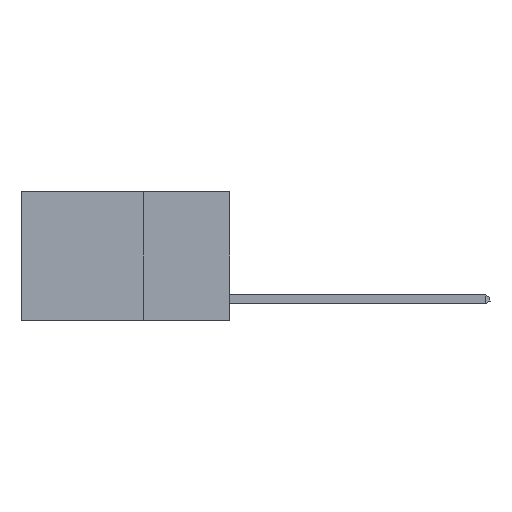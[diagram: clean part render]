
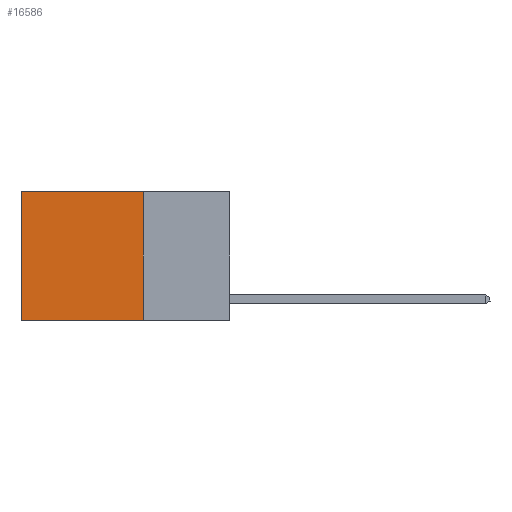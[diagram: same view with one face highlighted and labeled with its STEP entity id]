
A CAD part, left-side view. The second image highlights one B-rep face of the part: STEP entity #16586.
In plain terms, the highlighted planar face has unit normal (-1, 0, 0).
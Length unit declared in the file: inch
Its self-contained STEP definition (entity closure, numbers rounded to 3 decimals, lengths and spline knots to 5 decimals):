
#429 = VECTOR ( 'NONE', #10084, 39.37008 ) ;
#1538 = CARTESIAN_POINT ( 'NONE',  ( 0.2625, 0.25, -0.37 ) ) ;
#2339 = VERTEX_POINT ( 'NONE', #7589 ) ;
#2735 = AXIS2_PLACEMENT_3D ( 'NONE', #7296, #7208, #12312 ) ;
#3095 = LINE ( 'NONE', #10648, #5318 ) ;
#3541 = EDGE_CURVE ( 'NONE', #4128, #12841, #11182, .T. ) ;
#4128 = VERTEX_POINT ( 'NONE', #5209 ) ;
#4761 = LINE ( 'NONE', #4850, #5899 ) ;
#4764 = FACE_OUTER_BOUND ( 'NONE', #12498, .T. ) ;
#4850 = CARTESIAN_POINT ( 'NONE',  ( 0.2625, 0.25, -0.37 ) ) ;
#4935 = DIRECTION ( 'NONE',  ( 0., 0., -1. ) ) ;
#5209 = CARTESIAN_POINT ( 'NONE',  ( 0.2625, 0.6, 0. ) ) ;
#5318 = VECTOR ( 'NONE', #11742, 39.37008 ) ;
#5486 = ORIENTED_EDGE ( 'NONE', *, *, #15442, .F. ) ;
#5899 = VECTOR ( 'NONE', #16595, 39.37008 ) ;
#6091 = CARTESIAN_POINT ( 'NONE',  ( 0.2625, 0.6, -0.37 ) ) ;
#7208 = DIRECTION ( 'NONE',  ( 1., 0., 0. ) ) ;
#7264 = VECTOR ( 'NONE', #4935, 39.37008 ) ;
#7296 = CARTESIAN_POINT ( 'NONE',  ( 0.2625, 0.25, 0. ) ) ;
#7589 = CARTESIAN_POINT ( 'NONE',  ( 0.2625, 0.25, 0. ) ) ;
#8354 = VERTEX_POINT ( 'NONE', #1538 ) ;
#8818 = ORIENTED_EDGE ( 'NONE', *, *, #11045, .T. ) ;
#9856 = LINE ( 'NONE', #13812, #7264 ) ;
#10084 = DIRECTION ( 'NONE',  ( 0., 0., -1. ) ) ;
#10648 = CARTESIAN_POINT ( 'NONE',  ( 0.2625, 0.25, 0. ) ) ;
#11045 = EDGE_CURVE ( 'NONE', #2339, #4128, #3095, .T. ) ;
#11182 = LINE ( 'NONE', #12122, #429 ) ;
#11742 = DIRECTION ( 'NONE',  ( 0., 1., 0. ) ) ;
#12051 = ORIENTED_EDGE ( 'NONE', *, *, #15356, .F. ) ;
#12122 = CARTESIAN_POINT ( 'NONE',  ( 0.2625, 0.6, 0. ) ) ;
#12312 = DIRECTION ( 'NONE',  ( 0., 0., -1. ) ) ;
#12498 = EDGE_LOOP ( 'NONE', ( #13303, #5486, #12051, #8818 ) ) ;
#12841 = VERTEX_POINT ( 'NONE', #6091 ) ;
#13303 = ORIENTED_EDGE ( 'NONE', *, *, #3541, .T. ) ;
#13317 = PLANE ( 'NONE',  #2735 ) ;
#13812 = CARTESIAN_POINT ( 'NONE',  ( 0.2625, 0.25, 0. ) ) ;
#15356 = EDGE_CURVE ( 'NONE', #2339, #8354, #9856, .T. ) ;
#15442 = EDGE_CURVE ( 'NONE', #8354, #12841, #4761, .T. ) ;
#16586 = ADVANCED_FACE ( 'NONE', ( #4764 ), #13317, .F. ) ;
#16595 = DIRECTION ( 'NONE',  ( 0., 1., 0. ) ) ;
